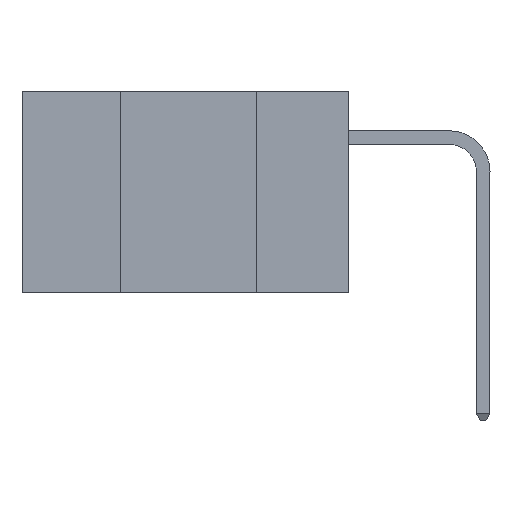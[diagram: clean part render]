
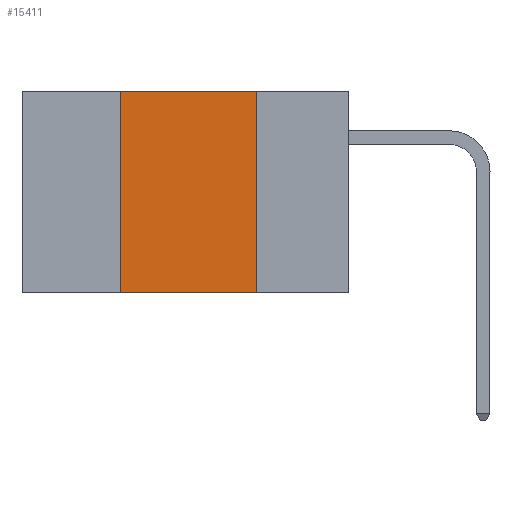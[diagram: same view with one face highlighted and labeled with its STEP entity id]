
A CAD part, left-side view. The second image highlights one B-rep face of the part: STEP entity #15411.
In plain terms, the highlighted planar face has unit normal (-1, 0, 0).
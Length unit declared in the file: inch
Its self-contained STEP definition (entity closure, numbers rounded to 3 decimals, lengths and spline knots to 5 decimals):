
#984 = VERTEX_POINT ( 'NONE', #25727 ) ;
#995 = LINE ( 'NONE', #6130, #13017 ) ;
#1279 = CARTESIAN_POINT ( 'NONE',  ( 0., 0.42, 0. ) ) ;
#1357 = DIRECTION ( 'NONE',  ( 0., 0., -1. ) ) ;
#2540 = CARTESIAN_POINT ( 'NONE',  ( 0., 0.42, -0.37 ) ) ;
#2932 = ORIENTED_EDGE ( 'NONE', *, *, #26398, .T. ) ;
#3629 = LINE ( 'NONE', #8162, #14819 ) ;
#4263 = VERTEX_POINT ( 'NONE', #8247 ) ;
#5619 = AXIS2_PLACEMENT_3D ( 'NONE', #29564, #15696, #1357 ) ;
#6130 = CARTESIAN_POINT ( 'NONE',  ( 0., 0.6, -0.37 ) ) ;
#6584 = EDGE_CURVE ( 'NONE', #984, #4263, #25790, .T. ) ;
#7270 = VERTEX_POINT ( 'NONE', #1279 ) ;
#8162 = CARTESIAN_POINT ( 'NONE',  ( 0., 0.42, 0. ) ) ;
#8247 = CARTESIAN_POINT ( 'NONE',  ( 0., 0.17, -0.37 ) ) ;
#8594 = PLANE ( 'NONE',  #5619 ) ;
#9571 = DIRECTION ( 'NONE',  ( 0., -1., 0. ) ) ;
#10701 = VECTOR ( 'NONE', #9571, 39.37008 ) ;
#12357 = CARTESIAN_POINT ( 'NONE',  ( 0., 0.17, 0. ) ) ;
#13017 = VECTOR ( 'NONE', #17864, 39.37008 ) ;
#14819 = VECTOR ( 'NONE', #15276, 39.37008 ) ;
#15276 = DIRECTION ( 'NONE',  ( 0., 0., 1. ) ) ;
#15411 = ADVANCED_FACE ( 'NONE', ( #20862 ), #8594, .F. ) ;
#15597 = ORIENTED_EDGE ( 'NONE', *, *, #6584, .F. ) ;
#15696 = DIRECTION ( 'NONE',  ( 1., 0., 0. ) ) ;
#17864 = DIRECTION ( 'NONE',  ( 0., -1., 0. ) ) ;
#19580 = VECTOR ( 'NONE', #26431, 39.37008 ) ;
#20155 = EDGE_CURVE ( 'NONE', #7270, #984, #23207, .T. ) ;
#20862 = FACE_OUTER_BOUND ( 'NONE', #25758, .T. ) ;
#23207 = LINE ( 'NONE', #28216, #10701 ) ;
#24758 = VERTEX_POINT ( 'NONE', #2540 ) ;
#25727 = CARTESIAN_POINT ( 'NONE',  ( 0., 0.17, 0. ) ) ;
#25758 = EDGE_LOOP ( 'NONE', ( #15597, #27619, #30477, #2932 ) ) ;
#25790 = LINE ( 'NONE', #12357, #19580 ) ;
#26398 = EDGE_CURVE ( 'NONE', #24758, #4263, #995, .T. ) ;
#26431 = DIRECTION ( 'NONE',  ( 0., 0., -1. ) ) ;
#26979 = EDGE_CURVE ( 'NONE', #24758, #7270, #3629, .T. ) ;
#27619 = ORIENTED_EDGE ( 'NONE', *, *, #20155, .F. ) ;
#28216 = CARTESIAN_POINT ( 'NONE',  ( 0., 0.6, 0. ) ) ;
#29564 = CARTESIAN_POINT ( 'NONE',  ( 0., 0.6, 0. ) ) ;
#30477 = ORIENTED_EDGE ( 'NONE', *, *, #26979, .F. ) ;
